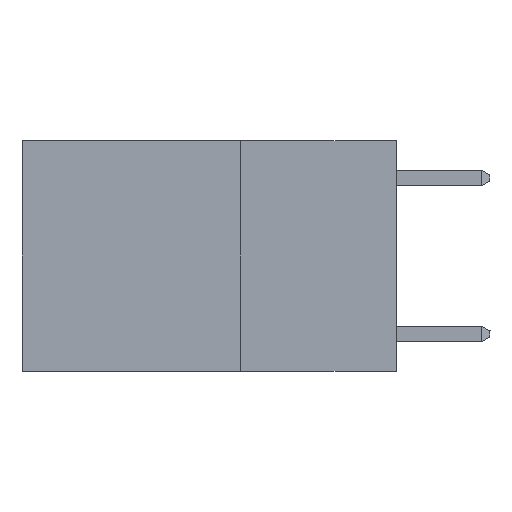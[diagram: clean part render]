
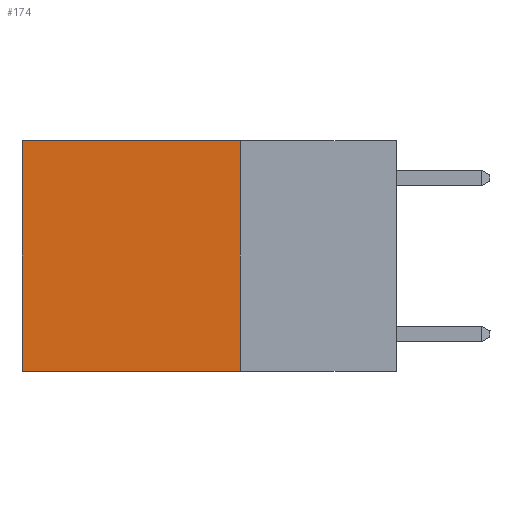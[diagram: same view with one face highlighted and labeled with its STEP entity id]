
A CAD part, left-side view. The second image highlights one B-rep face of the part: STEP entity #174.
In plain terms, the highlighted planar face has unit normal (-1, 0, 0).
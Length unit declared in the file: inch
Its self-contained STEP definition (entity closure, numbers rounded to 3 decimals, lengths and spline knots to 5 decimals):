
#174 = ADVANCED_FACE ( 'NONE', ( #14389 ), #14219, .F. ) ;
#1453 = EDGE_LOOP ( 'NONE', ( #3253, #15712, #16991, #10345 ) ) ;
#2302 = VERTEX_POINT ( 'NONE', #10632 ) ;
#3253 = ORIENTED_EDGE ( 'NONE', *, *, #9175, .T. ) ;
#5099 = LINE ( 'NONE', #15532, #12280 ) ;
#6027 = LINE ( 'NONE', #8404, #10123 ) ;
#6376 = DIRECTION ( 'NONE',  ( 0., 0., -1. ) ) ;
#6479 = VERTEX_POINT ( 'NONE', #13655 ) ;
#7505 = EDGE_CURVE ( 'NONE', #11896, #2302, #13963, .T. ) ;
#7726 = CARTESIAN_POINT ( 'NONE',  ( 0.2625, 0.25, -0.37 ) ) ;
#8160 = VECTOR ( 'NONE', #14304, 39.37008 ) ;
#8404 = CARTESIAN_POINT ( 'NONE',  ( 0.2625, 0.6, 0. ) ) ;
#8636 = AXIS2_PLACEMENT_3D ( 'NONE', #10471, #9186, #6376 ) ;
#9175 = EDGE_CURVE ( 'NONE', #14677, #2302, #6027, .T. ) ;
#9186 = DIRECTION ( 'NONE',  ( 1., 0., 0. ) ) ;
#9662 = CARTESIAN_POINT ( 'NONE',  ( 0.2625, 0.6, 0. ) ) ;
#9856 = CARTESIAN_POINT ( 'NONE',  ( 0.2625, 0.25, 0. ) ) ;
#10123 = VECTOR ( 'NONE', #16461, 39.37008 ) ;
#10125 = DIRECTION ( 'NONE',  ( 0., 0., -1. ) ) ;
#10345 = ORIENTED_EDGE ( 'NONE', *, *, #15663, .T. ) ;
#10471 = CARTESIAN_POINT ( 'NONE',  ( 0.2625, 0.25, 0. ) ) ;
#10488 = EDGE_CURVE ( 'NONE', #6479, #11896, #5099, .T. ) ;
#10632 = CARTESIAN_POINT ( 'NONE',  ( 0.2625, 0.6, -0.37 ) ) ;
#10974 = LINE ( 'NONE', #9856, #16353 ) ;
#11720 = CARTESIAN_POINT ( 'NONE',  ( 0.2625, 0.25, -0.37 ) ) ;
#11896 = VERTEX_POINT ( 'NONE', #11720 ) ;
#12280 = VECTOR ( 'NONE', #10125, 39.37008 ) ;
#13655 = CARTESIAN_POINT ( 'NONE',  ( 0.2625, 0.25, 0. ) ) ;
#13963 = LINE ( 'NONE', #7726, #8160 ) ;
#14219 = PLANE ( 'NONE',  #8636 ) ;
#14304 = DIRECTION ( 'NONE',  ( 0., 1., 0. ) ) ;
#14389 = FACE_OUTER_BOUND ( 'NONE', #1453, .T. ) ;
#14677 = VERTEX_POINT ( 'NONE', #9662 ) ;
#15532 = CARTESIAN_POINT ( 'NONE',  ( 0.2625, 0.25, 0. ) ) ;
#15663 = EDGE_CURVE ( 'NONE', #6479, #14677, #10974, .T. ) ;
#15712 = ORIENTED_EDGE ( 'NONE', *, *, #7505, .F. ) ;
#16353 = VECTOR ( 'NONE', #16371, 39.37008 ) ;
#16371 = DIRECTION ( 'NONE',  ( 0., 1., 0. ) ) ;
#16461 = DIRECTION ( 'NONE',  ( 0., 0., -1. ) ) ;
#16991 = ORIENTED_EDGE ( 'NONE', *, *, #10488, .F. ) ;
